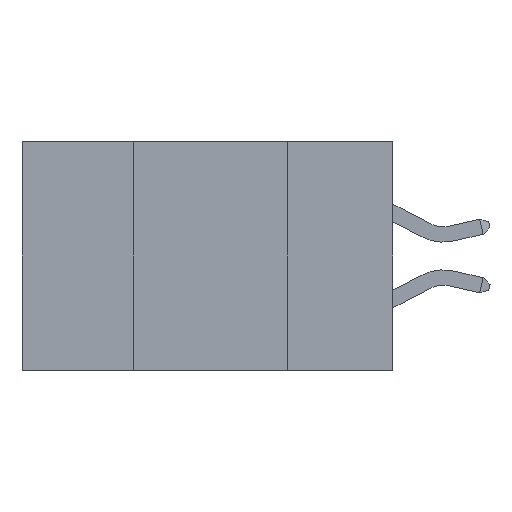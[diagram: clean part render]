
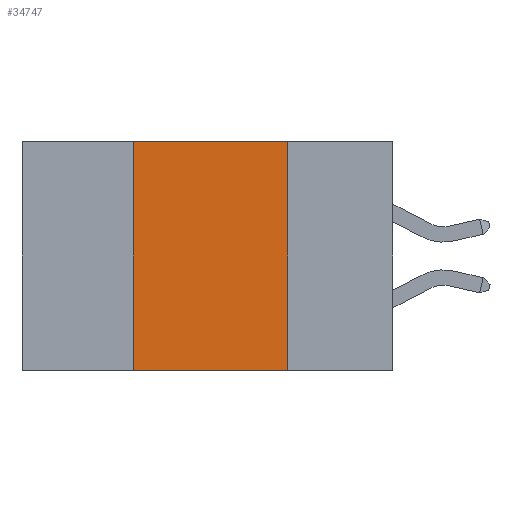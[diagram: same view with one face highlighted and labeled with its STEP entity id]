
A CAD part, left-side view. The second image highlights one B-rep face of the part: STEP entity #34747.
In plain terms, the highlighted planar face has unit normal (-1, 0, 0).
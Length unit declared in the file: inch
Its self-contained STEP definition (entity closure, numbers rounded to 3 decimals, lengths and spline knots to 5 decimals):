
#1373 = LINE ( 'NONE', #24826, #23763 ) ;
#1727 = CARTESIAN_POINT ( 'NONE',  ( 0., 0.42, -0.37 ) ) ;
#2525 = CARTESIAN_POINT ( 'NONE',  ( 0., 0.17, 0. ) ) ;
#2806 = DIRECTION ( 'NONE',  ( 1., 0., 0. ) ) ;
#5750 = LINE ( 'NONE', #30690, #29085 ) ;
#6013 = FACE_OUTER_BOUND ( 'NONE', #11916, .T. ) ;
#6341 = ORIENTED_EDGE ( 'NONE', *, *, #6539, .F. ) ;
#6539 = EDGE_CURVE ( 'NONE', #32101, #37823, #14760, .T. ) ;
#7005 = VECTOR ( 'NONE', #34459, 39.37008 ) ;
#7499 = ORIENTED_EDGE ( 'NONE', *, *, #9485, .T. ) ;
#9485 = EDGE_CURVE ( 'NONE', #24409, #37823, #1373, .T. ) ;
#10377 = DIRECTION ( 'NONE',  ( 0., -1., 0. ) ) ;
#11870 = DIRECTION ( 'NONE',  ( 0., 0., -1. ) ) ;
#11916 = EDGE_LOOP ( 'NONE', ( #6341, #17736, #30344, #7499 ) ) ;
#13219 = DIRECTION ( 'NONE',  ( 0., -1., 0. ) ) ;
#14265 = AXIS2_PLACEMENT_3D ( 'NONE', #37828, #2806, #11870 ) ;
#14447 = CARTESIAN_POINT ( 'NONE',  ( 0., 0.17, -0.37 ) ) ;
#14682 = EDGE_CURVE ( 'NONE', #24409, #22617, #20710, .T. ) ;
#14760 = LINE ( 'NONE', #2525, #7005 ) ;
#17736 = ORIENTED_EDGE ( 'NONE', *, *, #21527, .F. ) ;
#20169 = PLANE ( 'NONE',  #14265 ) ;
#20710 = LINE ( 'NONE', #31911, #37250 ) ;
#21527 = EDGE_CURVE ( 'NONE', #22617, #32101, #5750, .T. ) ;
#22617 = VERTEX_POINT ( 'NONE', #32115 ) ;
#23193 = CARTESIAN_POINT ( 'NONE',  ( 0., 0.17, 0. ) ) ;
#23763 = VECTOR ( 'NONE', #10377, 39.37008 ) ;
#24409 = VERTEX_POINT ( 'NONE', #1727 ) ;
#24826 = CARTESIAN_POINT ( 'NONE',  ( 0., 0.6, -0.37 ) ) ;
#26639 = DIRECTION ( 'NONE',  ( 0., 0., 1. ) ) ;
#29085 = VECTOR ( 'NONE', #13219, 39.37008 ) ;
#30344 = ORIENTED_EDGE ( 'NONE', *, *, #14682, .F. ) ;
#30690 = CARTESIAN_POINT ( 'NONE',  ( 0., 0.6, 0. ) ) ;
#31911 = CARTESIAN_POINT ( 'NONE',  ( 0., 0.42, 0. ) ) ;
#32101 = VERTEX_POINT ( 'NONE', #23193 ) ;
#32115 = CARTESIAN_POINT ( 'NONE',  ( 0., 0.42, 0. ) ) ;
#34459 = DIRECTION ( 'NONE',  ( 0., 0., -1. ) ) ;
#34747 = ADVANCED_FACE ( 'NONE', ( #6013 ), #20169, .F. ) ;
#37250 = VECTOR ( 'NONE', #26639, 39.37008 ) ;
#37823 = VERTEX_POINT ( 'NONE', #14447 ) ;
#37828 = CARTESIAN_POINT ( 'NONE',  ( 0., 0.6, 0. ) ) ;
